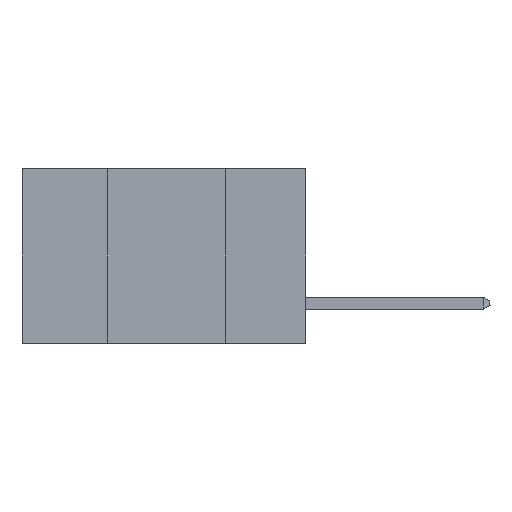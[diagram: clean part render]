
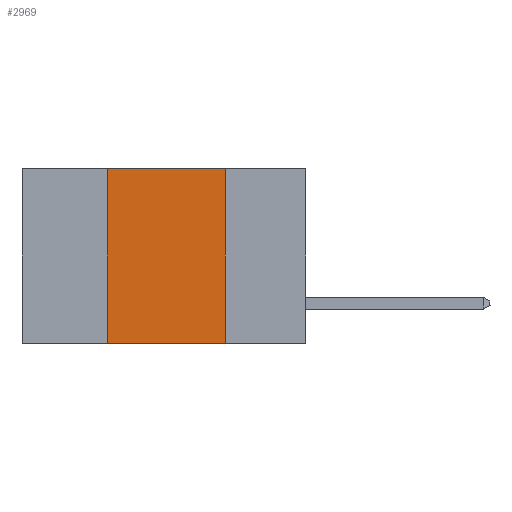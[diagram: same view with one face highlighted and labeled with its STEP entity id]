
A CAD part, left-side view. The second image highlights one B-rep face of the part: STEP entity #2969.
In plain terms, the highlighted planar face has unit normal (-1, 0, 0).
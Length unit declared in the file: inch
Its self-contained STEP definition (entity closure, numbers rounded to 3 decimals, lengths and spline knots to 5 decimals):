
#1442 = AXIS2_PLACEMENT_3D ( 'NONE', #12874, #2594, #14605 ) ;
#2048 = CARTESIAN_POINT ( 'NONE',  ( 0., 0.6, 0. ) ) ;
#2554 = VERTEX_POINT ( 'NONE', #16860 ) ;
#2594 = DIRECTION ( 'NONE',  ( 1., 0., 0. ) ) ;
#2622 = LINE ( 'NONE', #21404, #3941 ) ;
#2969 = ADVANCED_FACE ( 'NONE', ( #3338 ), #12806, .F. ) ;
#3054 = DIRECTION ( 'NONE',  ( 0., -1., 0. ) ) ;
#3338 = FACE_OUTER_BOUND ( 'NONE', #16452, .T. ) ;
#3941 = VECTOR ( 'NONE', #4519, 39.37008 ) ;
#4519 = DIRECTION ( 'NONE',  ( 0., 0., 1. ) ) ;
#4551 = VERTEX_POINT ( 'NONE', #10328 ) ;
#4852 = ORIENTED_EDGE ( 'NONE', *, *, #7257, .F. ) ;
#6137 = CARTESIAN_POINT ( 'NONE',  ( 0., 0.17, 0. ) ) ;
#6777 = LINE ( 'NONE', #21967, #18069 ) ;
#7257 = EDGE_CURVE ( 'NONE', #4551, #20776, #2622, .T. ) ;
#7440 = LINE ( 'NONE', #2048, #15514 ) ;
#7733 = ORIENTED_EDGE ( 'NONE', *, *, #8049, .T. ) ;
#8038 = VERTEX_POINT ( 'NONE', #6137 ) ;
#8049 = EDGE_CURVE ( 'NONE', #4551, #2554, #9836, .T. ) ;
#9115 = ORIENTED_EDGE ( 'NONE', *, *, #20255, .F. ) ;
#9795 = DIRECTION ( 'NONE',  ( 0., 0., -1. ) ) ;
#9836 = LINE ( 'NONE', #10249, #21091 ) ;
#10249 = CARTESIAN_POINT ( 'NONE',  ( 0., 0.6, -0.37 ) ) ;
#10328 = CARTESIAN_POINT ( 'NONE',  ( 0., 0.42, -0.37 ) ) ;
#10511 = DIRECTION ( 'NONE',  ( 0., -1., 0. ) ) ;
#11485 = CARTESIAN_POINT ( 'NONE',  ( 0., 0.42, 0. ) ) ;
#12806 = PLANE ( 'NONE',  #1442 ) ;
#12874 = CARTESIAN_POINT ( 'NONE',  ( 0., 0.6, 0. ) ) ;
#14605 = DIRECTION ( 'NONE',  ( 0., 0., -1. ) ) ;
#15514 = VECTOR ( 'NONE', #10511, 39.37008 ) ;
#16452 = EDGE_LOOP ( 'NONE', ( #9115, #20510, #4852, #7733 ) ) ;
#16860 = CARTESIAN_POINT ( 'NONE',  ( 0., 0.17, -0.37 ) ) ;
#18069 = VECTOR ( 'NONE', #9795, 39.37008 ) ;
#18306 = EDGE_CURVE ( 'NONE', #20776, #8038, #7440, .T. ) ;
#20255 = EDGE_CURVE ( 'NONE', #8038, #2554, #6777, .T. ) ;
#20510 = ORIENTED_EDGE ( 'NONE', *, *, #18306, .F. ) ;
#20776 = VERTEX_POINT ( 'NONE', #11485 ) ;
#21091 = VECTOR ( 'NONE', #3054, 39.37008 ) ;
#21404 = CARTESIAN_POINT ( 'NONE',  ( 0., 0.42, 0. ) ) ;
#21967 = CARTESIAN_POINT ( 'NONE',  ( 0., 0.17, 0. ) ) ;
